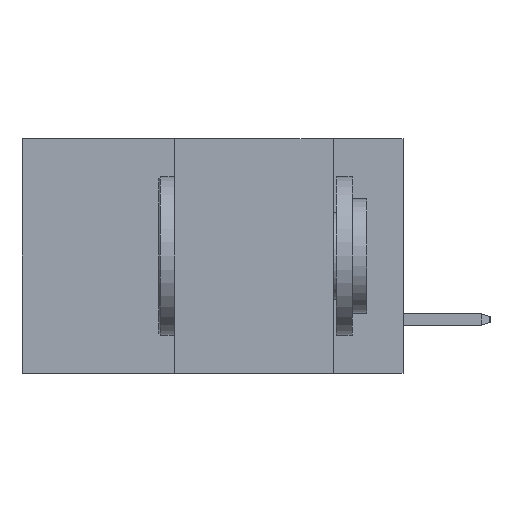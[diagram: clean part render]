
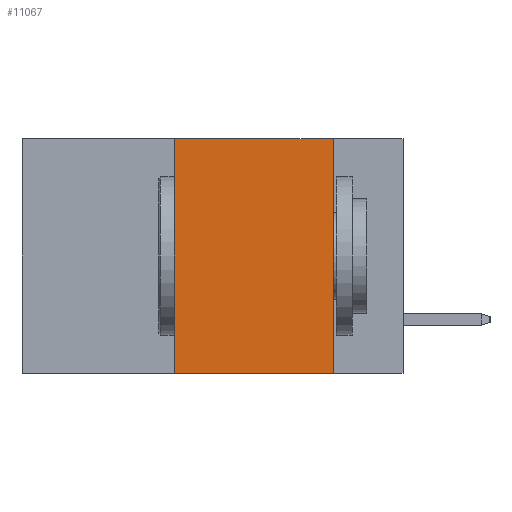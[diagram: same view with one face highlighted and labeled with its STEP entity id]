
A CAD part, left-side view. The second image highlights one B-rep face of the part: STEP entity #11067.
In plain terms, the highlighted planar face has unit normal (-1, 0, 0).
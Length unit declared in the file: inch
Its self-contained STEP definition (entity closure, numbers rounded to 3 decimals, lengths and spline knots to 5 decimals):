
#191 = DIRECTION ( 'NONE',  ( 0., 0., 1. ) ) ;
#549 = VERTEX_POINT ( 'NONE', #11448 ) ;
#888 = DIRECTION ( 'NONE',  ( 0., -1., 0. ) ) ;
#1120 = EDGE_CURVE ( 'NONE', #549, #13661, #12225, .T. ) ;
#2019 = VERTEX_POINT ( 'NONE', #16077 ) ;
#2461 = CARTESIAN_POINT ( 'NONE',  ( 0., 0.6, -0.37 ) ) ;
#2722 = DIRECTION ( 'NONE',  ( 0., 0., -1. ) ) ;
#3595 = ORIENTED_EDGE ( 'NONE', *, *, #10251, .F. ) ;
#4360 = LINE ( 'NONE', #10391, #10176 ) ;
#4663 = ORIENTED_EDGE ( 'NONE', *, *, #13935, .F. ) ;
#5035 = VERTEX_POINT ( 'NONE', #8448 ) ;
#5313 = VECTOR ( 'NONE', #15042, 39.37008 ) ;
#5383 = LINE ( 'NONE', #16910, #8534 ) ;
#8066 = DIRECTION ( 'NONE',  ( 1., 0., 0. ) ) ;
#8324 = VECTOR ( 'NONE', #888, 39.37008 ) ;
#8448 = CARTESIAN_POINT ( 'NONE',  ( 0., 0.11, 0. ) ) ;
#8534 = VECTOR ( 'NONE', #10986, 39.37008 ) ;
#10176 = VECTOR ( 'NONE', #191, 39.37008 ) ;
#10190 = AXIS2_PLACEMENT_3D ( 'NONE', #15349, #8066, #2722 ) ;
#10251 = EDGE_CURVE ( 'NONE', #549, #2019, #4360, .T. ) ;
#10391 = CARTESIAN_POINT ( 'NONE',  ( 0., 0.36, 0. ) ) ;
#10523 = LINE ( 'NONE', #17748, #5313 ) ;
#10652 = ORIENTED_EDGE ( 'NONE', *, *, #15410, .F. ) ;
#10986 = DIRECTION ( 'NONE',  ( 0., -1., 0. ) ) ;
#11067 = ADVANCED_FACE ( 'NONE', ( #15069 ), #16556, .F. ) ;
#11448 = CARTESIAN_POINT ( 'NONE',  ( 0., 0.36, -0.37 ) ) ;
#11963 = ORIENTED_EDGE ( 'NONE', *, *, #1120, .T. ) ;
#12225 = LINE ( 'NONE', #2461, #8324 ) ;
#13661 = VERTEX_POINT ( 'NONE', #14127 ) ;
#13935 = EDGE_CURVE ( 'NONE', #5035, #13661, #10523, .T. ) ;
#14127 = CARTESIAN_POINT ( 'NONE',  ( 0., 0.11, -0.37 ) ) ;
#14947 = EDGE_LOOP ( 'NONE', ( #4663, #10652, #3595, #11963 ) ) ;
#15042 = DIRECTION ( 'NONE',  ( 0., 0., -1. ) ) ;
#15069 = FACE_OUTER_BOUND ( 'NONE', #14947, .T. ) ;
#15349 = CARTESIAN_POINT ( 'NONE',  ( 0., 0.6, 0. ) ) ;
#15410 = EDGE_CURVE ( 'NONE', #2019, #5035, #5383, .T. ) ;
#16077 = CARTESIAN_POINT ( 'NONE',  ( 0., 0.36, 0. ) ) ;
#16556 = PLANE ( 'NONE',  #10190 ) ;
#16910 = CARTESIAN_POINT ( 'NONE',  ( 0., 0.6, 0. ) ) ;
#17748 = CARTESIAN_POINT ( 'NONE',  ( 0., 0.11, 0. ) ) ;
